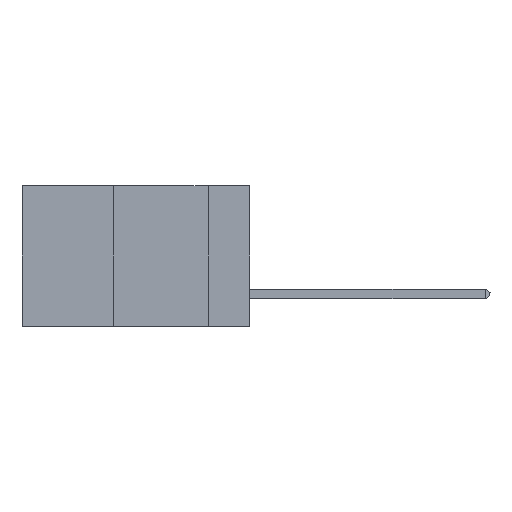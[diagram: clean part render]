
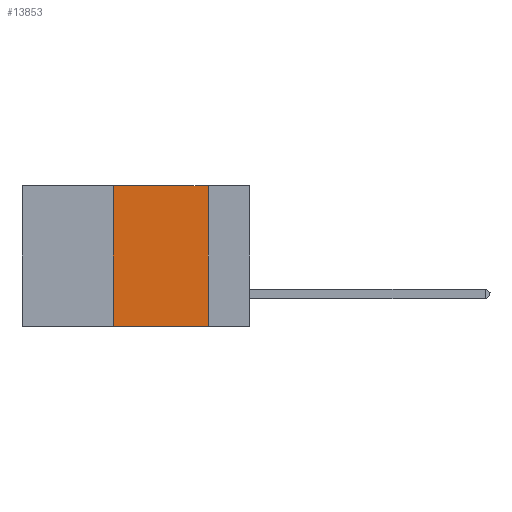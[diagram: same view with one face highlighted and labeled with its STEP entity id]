
A CAD part, left-side view. The second image highlights one B-rep face of the part: STEP entity #13853.
In plain terms, the highlighted planar face has unit normal (-1, 0, 0).
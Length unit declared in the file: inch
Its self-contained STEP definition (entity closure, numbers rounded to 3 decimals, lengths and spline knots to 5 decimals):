
#46 = VERTEX_POINT ( 'NONE', #8402 ) ;
#66 = EDGE_CURVE ( 'NONE', #46, #14654, #18415, .T. ) ;
#868 = LINE ( 'NONE', #886, #8128 ) ;
#886 = CARTESIAN_POINT ( 'NONE',  ( 0., 0.6, 0. ) ) ;
#1445 = LINE ( 'NONE', #3624, #6195 ) ;
#1686 = CARTESIAN_POINT ( 'NONE',  ( 0., 0.36, 0. ) ) ;
#3115 = ORIENTED_EDGE ( 'NONE', *, *, #6942, .F. ) ;
#3299 = VERTEX_POINT ( 'NONE', #1686 ) ;
#3623 = EDGE_LOOP ( 'NONE', ( #3115, #9613, #17065, #7720 ) ) ;
#3624 = CARTESIAN_POINT ( 'NONE',  ( 0., 0.11, 0. ) ) ;
#5180 = DIRECTION ( 'NONE',  ( 0., 0., -1. ) ) ;
#6078 = VECTOR ( 'NONE', #18789, 39.37008 ) ;
#6195 = VECTOR ( 'NONE', #5180, 39.37008 ) ;
#6734 = CARTESIAN_POINT ( 'NONE',  ( 0., 0.11, -0.37 ) ) ;
#6942 = EDGE_CURVE ( 'NONE', #15536, #14654, #1445, .T. ) ;
#7413 = CARTESIAN_POINT ( 'NONE',  ( 0., 0.11, 0. ) ) ;
#7720 = ORIENTED_EDGE ( 'NONE', *, *, #66, .T. ) ;
#8037 = AXIS2_PLACEMENT_3D ( 'NONE', #18338, #12571, #12449 ) ;
#8079 = PLANE ( 'NONE',  #8037 ) ;
#8128 = VECTOR ( 'NONE', #11045, 39.37008 ) ;
#8402 = CARTESIAN_POINT ( 'NONE',  ( 0., 0.36, -0.37 ) ) ;
#8730 = CARTESIAN_POINT ( 'NONE',  ( 0., 0.36, 0. ) ) ;
#9613 = ORIENTED_EDGE ( 'NONE', *, *, #10497, .F. ) ;
#10497 = EDGE_CURVE ( 'NONE', #3299, #15536, #868, .T. ) ;
#10731 = VECTOR ( 'NONE', #11656, 39.37008 ) ;
#11045 = DIRECTION ( 'NONE',  ( 0., -1., 0. ) ) ;
#11656 = DIRECTION ( 'NONE',  ( 0., -1., 0. ) ) ;
#11744 = EDGE_CURVE ( 'NONE', #46, #3299, #13798, .T. ) ;
#12449 = DIRECTION ( 'NONE',  ( 0., 0., -1. ) ) ;
#12571 = DIRECTION ( 'NONE',  ( 1., 0., 0. ) ) ;
#13798 = LINE ( 'NONE', #8730, #6078 ) ;
#13853 = ADVANCED_FACE ( 'NONE', ( #17417 ), #8079, .F. ) ;
#14654 = VERTEX_POINT ( 'NONE', #6734 ) ;
#15536 = VERTEX_POINT ( 'NONE', #7413 ) ;
#15596 = CARTESIAN_POINT ( 'NONE',  ( 0., 0.6, -0.37 ) ) ;
#17065 = ORIENTED_EDGE ( 'NONE', *, *, #11744, .F. ) ;
#17417 = FACE_OUTER_BOUND ( 'NONE', #3623, .T. ) ;
#18338 = CARTESIAN_POINT ( 'NONE',  ( 0., 0.6, 0. ) ) ;
#18415 = LINE ( 'NONE', #15596, #10731 ) ;
#18789 = DIRECTION ( 'NONE',  ( 0., 0., 1. ) ) ;
